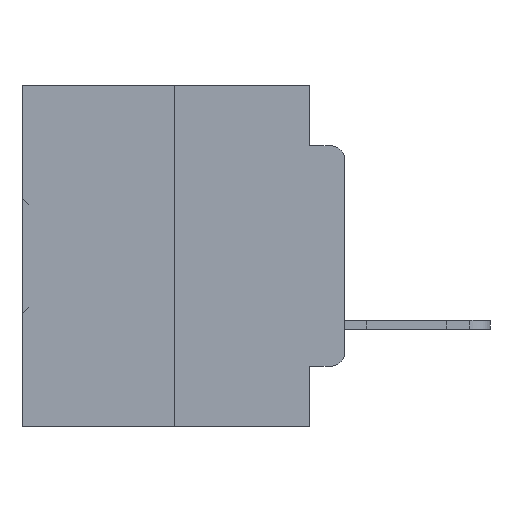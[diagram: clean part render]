
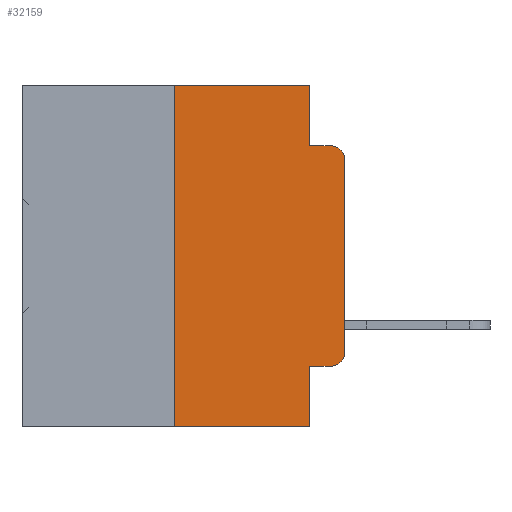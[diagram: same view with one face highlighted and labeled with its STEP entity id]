
A CAD part, left-side view. The second image highlights one B-rep face of the part: STEP entity #32159.
In plain terms, the highlighted planar face has unit normal (-1, 0, 0).
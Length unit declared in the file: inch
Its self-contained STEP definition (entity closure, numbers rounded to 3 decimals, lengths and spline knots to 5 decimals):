
#1084 = EDGE_CURVE ( 'NONE', #26368, #19333, #17851, .T. ) ;
#1331 = ORIENTED_EDGE ( 'NONE', *, *, #36123, .F. ) ;
#1885 = VECTOR ( 'NONE', #32986, 39.37008 ) ;
#1894 = CARTESIAN_POINT ( 'NONE',  ( 0., 0.25, 0. ) ) ;
#2246 = VECTOR ( 'NONE', #22789, 39.37008 ) ;
#2381 = VECTOR ( 'NONE', #35281, 39.37008 ) ;
#2872 = LINE ( 'NONE', #16148, #1885 ) ;
#2941 = LINE ( 'NONE', #4937, #32796 ) ;
#2984 = AXIS2_PLACEMENT_3D ( 'NONE', #14514, #34158, #17524 ) ;
#4149 = ORIENTED_EDGE ( 'NONE', *, *, #23389, .F. ) ;
#4494 = DIRECTION ( 'NONE',  ( 0., 0., -1. ) ) ;
#4937 = CARTESIAN_POINT ( 'NONE',  ( 0., 0.051, -0.0885 ) ) ;
#6482 = DIRECTION ( 'NONE',  ( 0., 0., -1. ) ) ;
#6533 = DIRECTION ( 'NONE',  ( -1., 0., 0. ) ) ;
#6570 = CARTESIAN_POINT ( 'NONE',  ( 0., 0.051, 0. ) ) ;
#6579 = CARTESIAN_POINT ( 'NONE',  ( 0., 0.02, -0.3915 ) ) ;
#6654 = ORIENTED_EDGE ( 'NONE', *, *, #36013, .T. ) ;
#6808 = LINE ( 'NONE', #30726, #21624 ) ;
#6884 = ORIENTED_EDGE ( 'NONE', *, *, #1084, .T. ) ;
#7055 = ORIENTED_EDGE ( 'NONE', *, *, #21448, .F. ) ;
#7377 = VERTEX_POINT ( 'NONE', #22208 ) ;
#7599 = EDGE_CURVE ( 'NONE', #9113, #18137, #10649, .T. ) ;
#7927 = CARTESIAN_POINT ( 'NONE',  ( 0., 0.051, -0.5 ) ) ;
#8029 = ORIENTED_EDGE ( 'NONE', *, *, #30678, .T. ) ;
#8154 = CIRCLE ( 'NONE', #2984, 0.02 ) ;
#9052 = VECTOR ( 'NONE', #36953, 39.37008 ) ;
#9113 = VERTEX_POINT ( 'NONE', #28165 ) ;
#9180 = ORIENTED_EDGE ( 'NONE', *, *, #17552, .T. ) ;
#9477 = ORIENTED_EDGE ( 'NONE', *, *, #7599, .T. ) ;
#9539 = DIRECTION ( 'NONE',  ( 1., 0., 0. ) ) ;
#10478 = LINE ( 'NONE', #1894, #2246 ) ;
#10514 = EDGE_LOOP ( 'NONE', ( #6654, #8029, #15876, #14890, #1331, #4149, #6884, #7055, #9180, #9477 ) ) ;
#10649 = CIRCLE ( 'NONE', #17802, 0.02 ) ;
#11131 = DIRECTION ( 'NONE',  ( 0., -1., 0. ) ) ;
#12895 = CARTESIAN_POINT ( 'NONE',  ( 0., 0.051, -0.0885 ) ) ;
#14514 = CARTESIAN_POINT ( 'NONE',  ( 0., 0.02, -0.1085 ) ) ;
#14890 = ORIENTED_EDGE ( 'NONE', *, *, #27005, .F. ) ;
#15646 = VERTEX_POINT ( 'NONE', #28059 ) ;
#15876 = ORIENTED_EDGE ( 'NONE', *, *, #28860, .F. ) ;
#16148 = CARTESIAN_POINT ( 'NONE',  ( 0., 0., 0. ) ) ;
#16265 = FACE_OUTER_BOUND ( 'NONE', #10514, .T. ) ;
#17086 = CARTESIAN_POINT ( 'NONE',  ( 0., 0.473, -0.5 ) ) ;
#17128 = VERTEX_POINT ( 'NONE', #12895 ) ;
#17472 = LINE ( 'NONE', #35876, #2381 ) ;
#17524 = DIRECTION ( 'NONE',  ( 0., 0., -1. ) ) ;
#17552 = EDGE_CURVE ( 'NONE', #7377, #9113, #17472, .T. ) ;
#17802 = AXIS2_PLACEMENT_3D ( 'NONE', #6579, #6533, #6482 ) ;
#17851 = LINE ( 'NONE', #17086, #9052 ) ;
#18137 = VERTEX_POINT ( 'NONE', #34419 ) ;
#19333 = VERTEX_POINT ( 'NONE', #7927 ) ;
#19371 = VERTEX_POINT ( 'NONE', #6570 ) ;
#21448 = EDGE_CURVE ( 'NONE', #7377, #19333, #33207, .T. ) ;
#21624 = VECTOR ( 'NONE', #22575, 39.37008 ) ;
#22208 = CARTESIAN_POINT ( 'NONE',  ( 0., 0.051, -0.4115 ) ) ;
#22575 = DIRECTION ( 'NONE',  ( 0., -1., 0. ) ) ;
#22789 = DIRECTION ( 'NONE',  ( 0., 0., 1. ) ) ;
#23389 = EDGE_CURVE ( 'NONE', #26368, #32842, #10478, .T. ) ;
#24092 = CARTESIAN_POINT ( 'NONE',  ( 0., 0.473, 0. ) ) ;
#24229 = CARTESIAN_POINT ( 'NONE',  ( 0., 0.02, -0.0885 ) ) ;
#24378 = VERTEX_POINT ( 'NONE', #24229 ) ;
#25901 = CARTESIAN_POINT ( 'NONE',  ( 0., 0.051, 0. ) ) ;
#26368 = VERTEX_POINT ( 'NONE', #34464 ) ;
#26580 = VECTOR ( 'NONE', #31243, 39.37008 ) ;
#27005 = EDGE_CURVE ( 'NONE', #19371, #17128, #30297, .T. ) ;
#28059 = CARTESIAN_POINT ( 'NONE',  ( 0., 0., -0.1085 ) ) ;
#28165 = CARTESIAN_POINT ( 'NONE',  ( 0., 0.02, -0.4115 ) ) ;
#28860 = EDGE_CURVE ( 'NONE', #17128, #24378, #2941, .T. ) ;
#29561 = DIRECTION ( 'NONE',  ( 0., 0., -1. ) ) ;
#30297 = LINE ( 'NONE', #25901, #26580 ) ;
#30678 = EDGE_CURVE ( 'NONE', #15646, #24378, #8154, .T. ) ;
#30726 = CARTESIAN_POINT ( 'NONE',  ( 0., 0.473, 0. ) ) ;
#31243 = DIRECTION ( 'NONE',  ( 0., 0., -1. ) ) ;
#32159 = ADVANCED_FACE ( 'NONE', ( #16265 ), #34841, .F. ) ;
#32361 = VECTOR ( 'NONE', #4494, 39.37008 ) ;
#32796 = VECTOR ( 'NONE', #11131, 39.37008 ) ;
#32824 = AXIS2_PLACEMENT_3D ( 'NONE', #24092, #9539, #29561 ) ;
#32842 = VERTEX_POINT ( 'NONE', #33153 ) ;
#32986 = DIRECTION ( 'NONE',  ( 0., 0., 1. ) ) ;
#33153 = CARTESIAN_POINT ( 'NONE',  ( 0., 0.25, 0. ) ) ;
#33207 = LINE ( 'NONE', #33307, #32361 ) ;
#33307 = CARTESIAN_POINT ( 'NONE',  ( 0., 0.051, 0. ) ) ;
#34158 = DIRECTION ( 'NONE',  ( -1., 0., 0. ) ) ;
#34419 = CARTESIAN_POINT ( 'NONE',  ( 0., 0., -0.3915 ) ) ;
#34464 = CARTESIAN_POINT ( 'NONE',  ( 0., 0.25, -0.5 ) ) ;
#34841 = PLANE ( 'NONE',  #32824 ) ;
#35281 = DIRECTION ( 'NONE',  ( 0., -1., 0. ) ) ;
#35876 = CARTESIAN_POINT ( 'NONE',  ( 0., 0.051, -0.4115 ) ) ;
#36013 = EDGE_CURVE ( 'NONE', #18137, #15646, #2872, .T. ) ;
#36123 = EDGE_CURVE ( 'NONE', #32842, #19371, #6808, .T. ) ;
#36953 = DIRECTION ( 'NONE',  ( 0., -1., 0. ) ) ;
